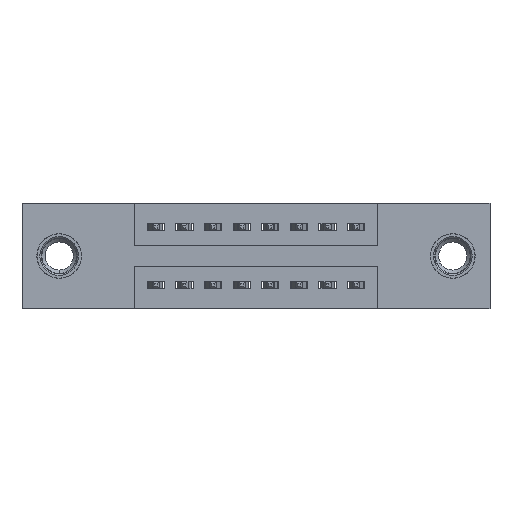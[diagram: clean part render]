
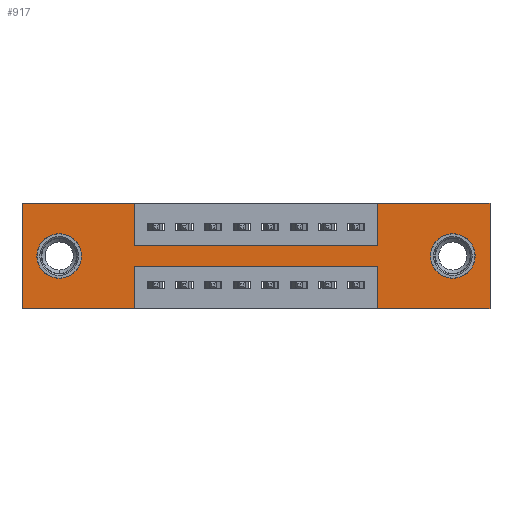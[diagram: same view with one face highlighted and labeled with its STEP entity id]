
A CAD part, front view. The second image highlights one B-rep face of the part: STEP entity #917.
In plain terms, the highlighted planar face has unit normal (0, -1, 0).
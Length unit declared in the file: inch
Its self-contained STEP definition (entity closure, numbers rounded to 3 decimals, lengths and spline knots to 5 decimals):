
#85 = VERTEX_POINT ( 'NONE', #2747 ) ;
#353 = VECTOR ( 'NONE', #2129, 39.37008 ) ;
#412 = VERTEX_POINT ( 'NONE', #5306 ) ;
#574 = EDGE_LOOP ( 'NONE', ( #11824, #5376 ) ) ;
#594 = CARTESIAN_POINT ( 'NONE',  ( 1.2425, 0., -0.37 ) ) ;
#785 = VERTEX_POINT ( 'NONE', #11234 ) ;
#887 = VECTOR ( 'NONE', #5633, 39.37008 ) ;
#897 = ORIENTED_EDGE ( 'NONE', *, *, #9821, .F. ) ;
#917 = ADVANCED_FACE ( 'NONE', ( #2056, #11679, #7014 ), #1938, .T. ) ;
#949 = CARTESIAN_POINT ( 'NONE',  ( 1.2425, 0., -0.15 ) ) ;
#1065 = VERTEX_POINT ( 'NONE', #10730 ) ;
#1205 = EDGE_CURVE ( 'NONE', #4791, #11836, #3869, .T. ) ;
#1400 = ORIENTED_EDGE ( 'NONE', *, *, #6885, .F. ) ;
#1411 = EDGE_CURVE ( 'NONE', #11273, #5030, #6475, .T. ) ;
#1429 = EDGE_LOOP ( 'NONE', ( #3267, #5788, #897, #8620, #7124, #9434, #2511, #5403, #10547, #1400, #11093, #11378 ) ) ;
#1504 = CARTESIAN_POINT ( 'NONE',  ( 0., 0., 0. ) ) ;
#1527 = VERTEX_POINT ( 'NONE', #11373 ) ;
#1569 = DIRECTION ( 'NONE',  ( 0., 0., -1. ) ) ;
#1594 = AXIS2_PLACEMENT_3D ( 'NONE', #2237, #1954, #1920 ) ;
#1643 = VERTEX_POINT ( 'NONE', #949 ) ;
#1646 = DIRECTION ( 'NONE',  ( 0., 1., 0. ) ) ;
#1669 = CIRCLE ( 'NONE', #2636, 0.078 ) ;
#1813 = LINE ( 'NONE', #3206, #4124 ) ;
#1875 = LINE ( 'NONE', #2386, #6349 ) ;
#1920 = DIRECTION ( 'NONE',  ( 0., 0., 1. ) ) ;
#1938 = PLANE ( 'NONE',  #2112 ) ;
#1954 = DIRECTION ( 'NONE',  ( 0., 1., 0. ) ) ;
#2056 = FACE_BOUND ( 'NONE', #3780, .T. ) ;
#2112 = AXIS2_PLACEMENT_3D ( 'NONE', #12072, #12047, #1569 ) ;
#2129 = DIRECTION ( 'NONE',  ( 0., 0., 1. ) ) ;
#2197 = VECTOR ( 'NONE', #12001, 39.37008 ) ;
#2211 = VECTOR ( 'NONE', #6295, 39.37008 ) ;
#2237 = CARTESIAN_POINT ( 'NONE',  ( 0.13, 0., -0.185 ) ) ;
#2386 = CARTESIAN_POINT ( 'NONE',  ( 1.2425, 0., -0.37 ) ) ;
#2491 = VECTOR ( 'NONE', #8220, 39.37008 ) ;
#2511 = ORIENTED_EDGE ( 'NONE', *, *, #11619, .F. ) ;
#2537 = DIRECTION ( 'NONE',  ( 0., 0., -1. ) ) ;
#2582 = EDGE_CURVE ( 'NONE', #412, #85, #5337, .T. ) ;
#2636 = AXIS2_PLACEMENT_3D ( 'NONE', #4174, #10354, #5121 ) ;
#2747 = CARTESIAN_POINT ( 'NONE',  ( 0.3925, 0., -0.37 ) ) ;
#2936 = EDGE_CURVE ( 'NONE', #11836, #4791, #1669, .T. ) ;
#2971 = CARTESIAN_POINT ( 'NONE',  ( 1.635, 0., 0. ) ) ;
#3055 = CARTESIAN_POINT ( 'NONE',  ( 0., 0., -0.37 ) ) ;
#3122 = LINE ( 'NONE', #2971, #7672 ) ;
#3206 = CARTESIAN_POINT ( 'NONE',  ( 0., 0., -0.37 ) ) ;
#3267 = ORIENTED_EDGE ( 'NONE', *, *, #2582, .F. ) ;
#3448 = CARTESIAN_POINT ( 'NONE',  ( 0.3925, 0., -0.22 ) ) ;
#3746 = CARTESIAN_POINT ( 'NONE',  ( 0.3925, 0., -0.37 ) ) ;
#3780 = EDGE_LOOP ( 'NONE', ( #8640, #9448 ) ) ;
#3869 = CIRCLE ( 'NONE', #9790, 0.078 ) ;
#3927 = DIRECTION ( 'NONE',  ( 0., 0., -1. ) ) ;
#4124 = VECTOR ( 'NONE', #5125, 39.37008 ) ;
#4174 = CARTESIAN_POINT ( 'NONE',  ( 1.505, 0., -0.185 ) ) ;
#4272 = CARTESIAN_POINT ( 'NONE',  ( 1.505, 0., -0.107 ) ) ;
#4426 = DIRECTION ( 'NONE',  ( -1., 0., 0. ) ) ;
#4439 = CARTESIAN_POINT ( 'NONE',  ( 0.3925, 0., 0. ) ) ;
#4668 = CARTESIAN_POINT ( 'NONE',  ( 0.13, 0., -0.107 ) ) ;
#4743 = VERTEX_POINT ( 'NONE', #8607 ) ;
#4750 = EDGE_CURVE ( 'NONE', #85, #6590, #1813, .T. ) ;
#4791 = VERTEX_POINT ( 'NONE', #4272 ) ;
#4952 = CARTESIAN_POINT ( 'NONE',  ( 0.3925, 0., -0.15 ) ) ;
#5030 = VERTEX_POINT ( 'NONE', #4668 ) ;
#5121 = DIRECTION ( 'NONE',  ( 0., 0., -1. ) ) ;
#5125 = DIRECTION ( 'NONE',  ( -1., 0., 0. ) ) ;
#5306 = CARTESIAN_POINT ( 'NONE',  ( 0.3925, 0., -0.22 ) ) ;
#5337 = LINE ( 'NONE', #3746, #2491 ) ;
#5376 = ORIENTED_EDGE ( 'NONE', *, *, #1411, .T. ) ;
#5393 = CARTESIAN_POINT ( 'NONE',  ( 0., 0., 0. ) ) ;
#5403 = ORIENTED_EDGE ( 'NONE', *, *, #10198, .F. ) ;
#5448 = CARTESIAN_POINT ( 'NONE',  ( 1.635, 0., -0.37 ) ) ;
#5476 = VECTOR ( 'NONE', #2537, 39.37008 ) ;
#5611 = EDGE_CURVE ( 'NONE', #11984, #6974, #6405, .T. ) ;
#5633 = DIRECTION ( 'NONE',  ( 1., 0., 0. ) ) ;
#5718 = AXIS2_PLACEMENT_3D ( 'NONE', #7256, #1646, #8111 ) ;
#5763 = CARTESIAN_POINT ( 'NONE',  ( 1.635, 0., 0. ) ) ;
#5770 = EDGE_CURVE ( 'NONE', #1065, #412, #11434, .T. ) ;
#5788 = ORIENTED_EDGE ( 'NONE', *, *, #5770, .F. ) ;
#6142 = VERTEX_POINT ( 'NONE', #11153 ) ;
#6194 = CARTESIAN_POINT ( 'NONE',  ( 1.505, 0., -0.263 ) ) ;
#6295 = DIRECTION ( 'NONE',  ( 0., 0., 1. ) ) ;
#6349 = VECTOR ( 'NONE', #8761, 39.37008 ) ;
#6405 = LINE ( 'NONE', #10315, #10734 ) ;
#6475 = CIRCLE ( 'NONE', #1594, 0.078 ) ;
#6590 = VERTEX_POINT ( 'NONE', #3055 ) ;
#6782 = VECTOR ( 'NONE', #4426, 39.37008 ) ;
#6786 = CARTESIAN_POINT ( 'NONE',  ( 1.2425, 0., 0. ) ) ;
#6885 = EDGE_CURVE ( 'NONE', #4743, #1527, #10033, .T. ) ;
#6974 = VERTEX_POINT ( 'NONE', #594 ) ;
#7014 = FACE_OUTER_BOUND ( 'NONE', #1429, .T. ) ;
#7124 = ORIENTED_EDGE ( 'NONE', *, *, #8737, .F. ) ;
#7256 = CARTESIAN_POINT ( 'NONE',  ( 0.13, 0., -0.185 ) ) ;
#7672 = VECTOR ( 'NONE', #3927, 39.37008 ) ;
#7715 = VECTOR ( 'NONE', #11545, 39.37008 ) ;
#7867 = VERTEX_POINT ( 'NONE', #5763 ) ;
#8111 = DIRECTION ( 'NONE',  ( 0., 0., 1. ) ) ;
#8220 = DIRECTION ( 'NONE',  ( 0., 0., -1. ) ) ;
#8230 = CARTESIAN_POINT ( 'NONE',  ( 0., 0., 0. ) ) ;
#8349 = EDGE_CURVE ( 'NONE', #6590, #4743, #9186, .T. ) ;
#8447 = EDGE_CURVE ( 'NONE', #5030, #11273, #8636, .T. ) ;
#8451 = DIRECTION ( 'NONE',  ( 0., 0., -1. ) ) ;
#8607 = CARTESIAN_POINT ( 'NONE',  ( 0., 0., 0. ) ) ;
#8620 = ORIENTED_EDGE ( 'NONE', *, *, #5611, .F. ) ;
#8634 = DIRECTION ( 'NONE',  ( 0., 1., 0. ) ) ;
#8636 = CIRCLE ( 'NONE', #5718, 0.078 ) ;
#8640 = ORIENTED_EDGE ( 'NONE', *, *, #1205, .T. ) ;
#8651 = CARTESIAN_POINT ( 'NONE',  ( 1.505, 0., -0.185 ) ) ;
#8737 = EDGE_CURVE ( 'NONE', #7867, #11984, #3122, .T. ) ;
#8761 = DIRECTION ( 'NONE',  ( 0., 0., 1. ) ) ;
#9186 = LINE ( 'NONE', #5393, #2211 ) ;
#9434 = ORIENTED_EDGE ( 'NONE', *, *, #10834, .F. ) ;
#9448 = ORIENTED_EDGE ( 'NONE', *, *, #2936, .T. ) ;
#9790 = AXIS2_PLACEMENT_3D ( 'NONE', #8651, #8634, #8451 ) ;
#9821 = EDGE_CURVE ( 'NONE', #6974, #1065, #1875, .T. ) ;
#10033 = LINE ( 'NONE', #1504, #7715 ) ;
#10100 = LINE ( 'NONE', #4439, #5476 ) ;
#10198 = EDGE_CURVE ( 'NONE', #6142, #1643, #11807, .T. ) ;
#10315 = CARTESIAN_POINT ( 'NONE',  ( 0., 0., -0.37 ) ) ;
#10354 = DIRECTION ( 'NONE',  ( 0., 1., 0. ) ) ;
#10547 = ORIENTED_EDGE ( 'NONE', *, *, #11387, .F. ) ;
#10661 = LINE ( 'NONE', #8230, #887 ) ;
#10730 = CARTESIAN_POINT ( 'NONE',  ( 1.2425, 0., -0.22 ) ) ;
#10734 = VECTOR ( 'NONE', #11204, 39.37008 ) ;
#10781 = LINE ( 'NONE', #6786, #353 ) ;
#10834 = EDGE_CURVE ( 'NONE', #785, #7867, #10661, .T. ) ;
#11093 = ORIENTED_EDGE ( 'NONE', *, *, #8349, .F. ) ;
#11153 = CARTESIAN_POINT ( 'NONE',  ( 0.3925, 0., -0.15 ) ) ;
#11204 = DIRECTION ( 'NONE',  ( -1., 0., 0. ) ) ;
#11234 = CARTESIAN_POINT ( 'NONE',  ( 1.2425, 0., 0. ) ) ;
#11273 = VERTEX_POINT ( 'NONE', #11377 ) ;
#11373 = CARTESIAN_POINT ( 'NONE',  ( 0.3925, 0., 0. ) ) ;
#11377 = CARTESIAN_POINT ( 'NONE',  ( 0.13, 0., -0.263 ) ) ;
#11378 = ORIENTED_EDGE ( 'NONE', *, *, #4750, .F. ) ;
#11387 = EDGE_CURVE ( 'NONE', #1527, #6142, #10100, .T. ) ;
#11434 = LINE ( 'NONE', #3448, #6782 ) ;
#11545 = DIRECTION ( 'NONE',  ( 1., 0., 0. ) ) ;
#11619 = EDGE_CURVE ( 'NONE', #1643, #785, #10781, .T. ) ;
#11679 = FACE_BOUND ( 'NONE', #574, .T. ) ;
#11807 = LINE ( 'NONE', #4952, #2197 ) ;
#11824 = ORIENTED_EDGE ( 'NONE', *, *, #8447, .T. ) ;
#11836 = VERTEX_POINT ( 'NONE', #6194 ) ;
#11984 = VERTEX_POINT ( 'NONE', #5448 ) ;
#12001 = DIRECTION ( 'NONE',  ( 1., 0., 0. ) ) ;
#12047 = DIRECTION ( 'NONE',  ( 0., -1., 0. ) ) ;
#12072 = CARTESIAN_POINT ( 'NONE',  ( 0., 0., -0.37 ) ) ;
